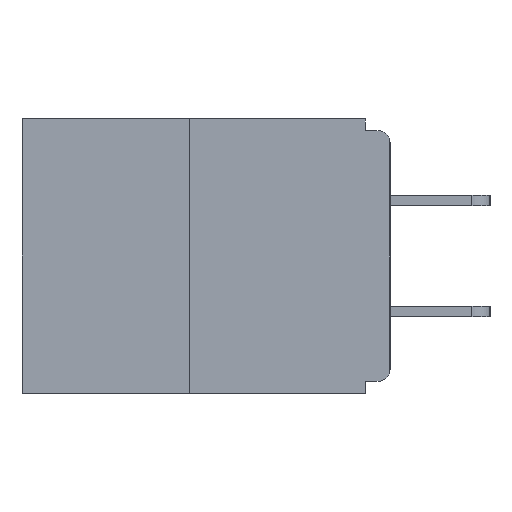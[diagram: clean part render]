
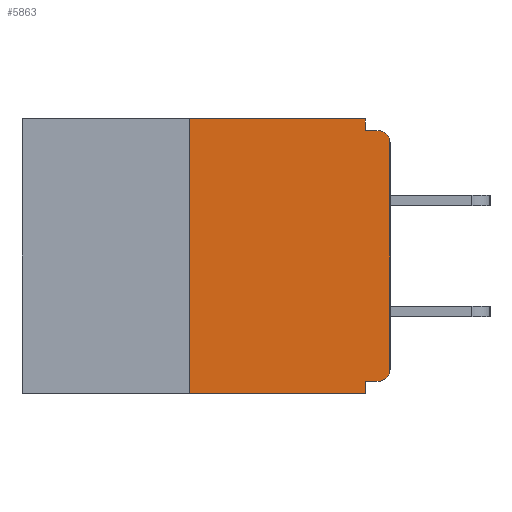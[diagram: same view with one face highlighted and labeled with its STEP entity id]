
A CAD part, left-side view. The second image highlights one B-rep face of the part: STEP entity #5863.
In plain terms, the highlighted planar face has unit normal (-1, 0, 0).
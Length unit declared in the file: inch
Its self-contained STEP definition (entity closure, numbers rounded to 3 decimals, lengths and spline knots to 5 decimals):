
#61 = VERTEX_POINT ( 'NONE', #3872 ) ;
#346 = EDGE_CURVE ( 'NONE', #12985, #10308, #10552, .T. ) ;
#1257 = DIRECTION ( 'NONE',  ( 0., 0., -1. ) ) ;
#1352 = CARTESIAN_POINT ( 'NONE',  ( 0., 0.25, -0.343 ) ) ;
#1433 = CIRCLE ( 'NONE', #16523, 0.015 ) ;
#2124 = PLANE ( 'NONE',  #7034 ) ;
#2555 = EDGE_CURVE ( 'NONE', #11193, #61, #3447, .T. ) ;
#2600 = LINE ( 'NONE', #10410, #3031 ) ;
#2823 = CARTESIAN_POINT ( 'NONE',  ( 0., 0.25, 0. ) ) ;
#3031 = VECTOR ( 'NONE', #15917, 39.37008 ) ;
#3057 = ORIENTED_EDGE ( 'NONE', *, *, #3807, .T. ) ;
#3332 = DIRECTION ( 'NONE',  ( 1., 0., 0. ) ) ;
#3447 = LINE ( 'NONE', #6336, #10796 ) ;
#3807 = EDGE_CURVE ( 'NONE', #12985, #61, #10095, .T. ) ;
#3872 = CARTESIAN_POINT ( 'NONE',  ( 0., 0.031, -0.343 ) ) ;
#4155 = CARTESIAN_POINT ( 'NONE',  ( 0., 0.015, -0.03 ) ) ;
#4506 = CARTESIAN_POINT ( 'NONE',  ( 0., 0.25, 0. ) ) ;
#4749 = ORIENTED_EDGE ( 'NONE', *, *, #346, .F. ) ;
#5562 = ORIENTED_EDGE ( 'NONE', *, *, #13742, .T. ) ;
#5591 = VERTEX_POINT ( 'NONE', #11716 ) ;
#5722 = CARTESIAN_POINT ( 'NONE',  ( 0., 0., -0.328 ) ) ;
#5863 = ADVANCED_FACE ( 'NONE', ( #16081 ), #2124, .F. ) ;
#6228 = CARTESIAN_POINT ( 'NONE',  ( 0., 0.46, 0. ) ) ;
#6281 = CARTESIAN_POINT ( 'NONE',  ( 0., 0., 0. ) ) ;
#6336 = CARTESIAN_POINT ( 'NONE',  ( 0., 0.031, -0.343 ) ) ;
#6728 = VERTEX_POINT ( 'NONE', #14272 ) ;
#6879 = DIRECTION ( 'NONE',  ( 0., -1., 0. ) ) ;
#7000 = EDGE_LOOP ( 'NONE', ( #7209, #4749, #3057, #7389, #15227, #7899, #14970, #5562, #8702, #10556 ) ) ;
#7034 = AXIS2_PLACEMENT_3D ( 'NONE', #6228, #3332, #17177 ) ;
#7110 = CARTESIAN_POINT ( 'NONE',  ( 0., 0.031, -0.015 ) ) ;
#7209 = ORIENTED_EDGE ( 'NONE', *, *, #17514, .F. ) ;
#7374 = VERTEX_POINT ( 'NONE', #12007 ) ;
#7389 = ORIENTED_EDGE ( 'NONE', *, *, #2555, .F. ) ;
#7590 = CARTESIAN_POINT ( 'NONE',  ( 0., 0.015, -0.313 ) ) ;
#7638 = LINE ( 'NONE', #6281, #14769 ) ;
#7899 = ORIENTED_EDGE ( 'NONE', *, *, #8993, .T. ) ;
#8702 = ORIENTED_EDGE ( 'NONE', *, *, #11067, .F. ) ;
#8993 = EDGE_CURVE ( 'NONE', #5591, #17125, #12169, .T. ) ;
#9034 = EDGE_CURVE ( 'NONE', #6728, #17639, #12602, .T. ) ;
#9493 = EDGE_CURVE ( 'NONE', #17125, #17604, #7638, .T. ) ;
#10095 = LINE ( 'NONE', #15165, #15507 ) ;
#10308 = VERTEX_POINT ( 'NONE', #4506 ) ;
#10410 = CARTESIAN_POINT ( 'NONE',  ( 0., 0., -0.015 ) ) ;
#10439 = VECTOR ( 'NONE', #12933, 39.37008 ) ;
#10552 = LINE ( 'NONE', #2823, #17489 ) ;
#10556 = ORIENTED_EDGE ( 'NONE', *, *, #9034, .F. ) ;
#10636 = EDGE_CURVE ( 'NONE', #5591, #11193, #10804, .T. ) ;
#10796 = VECTOR ( 'NONE', #17408, 39.37008 ) ;
#10804 = LINE ( 'NONE', #5722, #14925 ) ;
#11067 = EDGE_CURVE ( 'NONE', #17639, #7374, #2600, .T. ) ;
#11193 = VERTEX_POINT ( 'NONE', #14794 ) ;
#11648 = DIRECTION ( 'NONE',  ( 0., 0., 1. ) ) ;
#11716 = CARTESIAN_POINT ( 'NONE',  ( 0., 0.015, -0.328 ) ) ;
#11729 = DIRECTION ( 'NONE',  ( -1., 0., 0. ) ) ;
#12007 = CARTESIAN_POINT ( 'NONE',  ( 0., 0.015, -0.015 ) ) ;
#12169 = CIRCLE ( 'NONE', #16480, 0.015 ) ;
#12602 = LINE ( 'NONE', #12878, #10439 ) ;
#12672 = DIRECTION ( 'NONE',  ( 0., 1., 0. ) ) ;
#12740 = DIRECTION ( 'NONE',  ( 0., 0., 1. ) ) ;
#12878 = CARTESIAN_POINT ( 'NONE',  ( 0., 0.031, 0. ) ) ;
#12933 = DIRECTION ( 'NONE',  ( 0., 0., -1. ) ) ;
#12985 = VERTEX_POINT ( 'NONE', #1352 ) ;
#12993 = DIRECTION ( 'NONE',  ( 0., 0., -1. ) ) ;
#13742 = EDGE_CURVE ( 'NONE', #17604, #7374, #1433, .T. ) ;
#13816 = DIRECTION ( 'NONE',  ( -1., 0., 0. ) ) ;
#14272 = CARTESIAN_POINT ( 'NONE',  ( 0., 0.031, 0. ) ) ;
#14769 = VECTOR ( 'NONE', #11648, 39.37008 ) ;
#14794 = CARTESIAN_POINT ( 'NONE',  ( 0., 0.031, -0.328 ) ) ;
#14925 = VECTOR ( 'NONE', #12672, 39.37008 ) ;
#14970 = ORIENTED_EDGE ( 'NONE', *, *, #9493, .T. ) ;
#14987 = LINE ( 'NONE', #16075, #17136 ) ;
#15162 = CARTESIAN_POINT ( 'NONE',  ( 0., 0., -0.03 ) ) ;
#15165 = CARTESIAN_POINT ( 'NONE',  ( 0., 0.46, -0.343 ) ) ;
#15227 = ORIENTED_EDGE ( 'NONE', *, *, #10636, .F. ) ;
#15425 = CARTESIAN_POINT ( 'NONE',  ( 0., 0., -0.313 ) ) ;
#15507 = VECTOR ( 'NONE', #6879, 39.37008 ) ;
#15917 = DIRECTION ( 'NONE',  ( 0., -1., 0. ) ) ;
#16075 = CARTESIAN_POINT ( 'NONE',  ( 0., 0.46, 0. ) ) ;
#16081 = FACE_OUTER_BOUND ( 'NONE', #7000, .T. ) ;
#16480 = AXIS2_PLACEMENT_3D ( 'NONE', #7590, #11729, #12993 ) ;
#16523 = AXIS2_PLACEMENT_3D ( 'NONE', #4155, #13816, #1257 ) ;
#17125 = VERTEX_POINT ( 'NONE', #15425 ) ;
#17136 = VECTOR ( 'NONE', #17655, 39.37008 ) ;
#17177 = DIRECTION ( 'NONE',  ( 0., 0., -1. ) ) ;
#17408 = DIRECTION ( 'NONE',  ( 0., 0., -1. ) ) ;
#17489 = VECTOR ( 'NONE', #12740, 39.37008 ) ;
#17514 = EDGE_CURVE ( 'NONE', #10308, #6728, #14987, .T. ) ;
#17604 = VERTEX_POINT ( 'NONE', #15162 ) ;
#17639 = VERTEX_POINT ( 'NONE', #7110 ) ;
#17655 = DIRECTION ( 'NONE',  ( 0., -1., 0. ) ) ;
